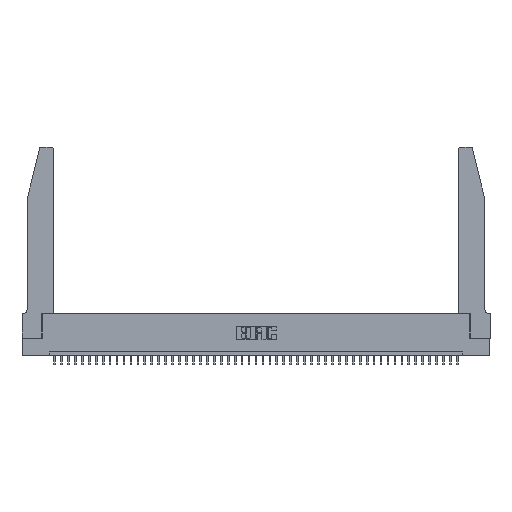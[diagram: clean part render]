
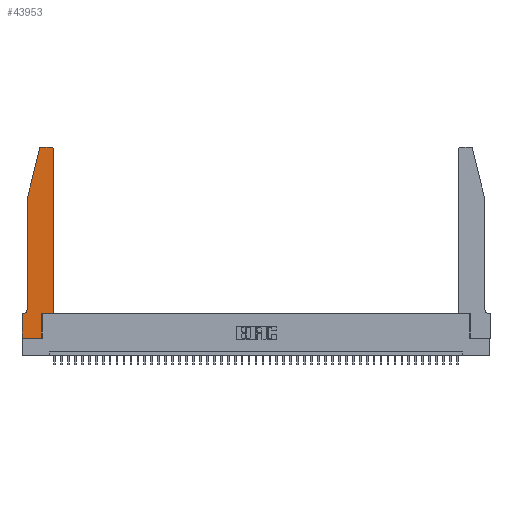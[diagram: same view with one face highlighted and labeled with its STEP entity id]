
A CAD part, top view. The second image highlights one B-rep face of the part: STEP entity #43953.
In plain terms, the highlighted planar face has unit normal (0, 0, 1).
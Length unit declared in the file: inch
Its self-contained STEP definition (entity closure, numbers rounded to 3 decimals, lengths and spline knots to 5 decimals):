
#138 = DIRECTION ( 'NONE',  ( -0.239, -0.971, 0. ) ) ;
#844 = DIRECTION ( 'NONE',  ( 1., 0., 0. ) ) ;
#2075 = VERTEX_POINT ( 'NONE', #14113 ) ;
#2103 = CARTESIAN_POINT ( 'NONE',  ( 0.284, 2.75, 0.37 ) ) ;
#2843 = VERTEX_POINT ( 'NONE', #15845 ) ;
#3227 = CARTESIAN_POINT ( 'NONE',  ( 0.4205, 2.72, 0.37 ) ) ;
#4551 = EDGE_CURVE ( 'NONE', #30048, #42664, #26186, .T. ) ;
#4882 = DIRECTION ( 'NONE',  ( 1., 0., 0. ) ) ;
#4928 = DIRECTION ( 'NONE',  ( 1., 0., 0. ) ) ;
#5244 = CARTESIAN_POINT ( 'NONE',  ( 0.2605, 2.75, 0.37 ) ) ;
#5633 = LINE ( 'NONE', #37370, #14106 ) ;
#5967 = VERTEX_POINT ( 'NONE', #39634 ) ;
#6289 = ORIENTED_EDGE ( 'NONE', *, *, #19652, .T. ) ;
#6685 = LINE ( 'NONE', #18117, #32146 ) ;
#7020 = EDGE_CURVE ( 'NONE', #42664, #39795, #6685, .T. ) ;
#8033 = CARTESIAN_POINT ( 'NONE',  ( 0.25487, 2.72718, 0.37 ) ) ;
#8486 = CARTESIAN_POINT ( 'NONE',  ( 0.0755, 2., 0.37 ) ) ;
#8851 = PLANE ( 'NONE',  #11352 ) ;
#10525 = EDGE_LOOP ( 'NONE', ( #17833, #34712, #24384, #11935, #15314, #38616, #31640, #6289, #16510, #16528, #33761, #29698 ) ) ;
#11204 = DIRECTION ( 'NONE',  ( -1., 0., 0. ) ) ;
#11352 = AXIS2_PLACEMENT_3D ( 'NONE', #44620, #30682, #4928 ) ;
#11652 = CIRCLE ( 'NONE', #34607, 0.07 ) ;
#11935 = ORIENTED_EDGE ( 'NONE', *, *, #13760, .T. ) ;
#12377 = LINE ( 'NONE', #18915, #35576 ) ;
#12575 = CARTESIAN_POINT ( 'NONE',  ( 0.0755, 0.42, 0.37 ) ) ;
#13193 = VERTEX_POINT ( 'NONE', #12575 ) ;
#13651 = DIRECTION ( 'NONE',  ( 1., 0., 0. ) ) ;
#13760 = EDGE_CURVE ( 'NONE', #39795, #13193, #5633, .T. ) ;
#14106 = VECTOR ( 'NONE', #18997, 39.37008 ) ;
#14113 = CARTESIAN_POINT ( 'NONE',  ( 0.4505, 0.35, 0.37 ) ) ;
#14118 = DIRECTION ( 'NONE',  ( 0., 0., 1. ) ) ;
#15143 = CARTESIAN_POINT ( 'NONE',  ( 0.0055, 0.42, 0.37 ) ) ;
#15176 = VECTOR ( 'NONE', #4882, 39.37008 ) ;
#15314 = ORIENTED_EDGE ( 'NONE', *, *, #15980, .T. ) ;
#15817 = VECTOR ( 'NONE', #844, 39.37008 ) ;
#15845 = CARTESIAN_POINT ( 'NONE',  ( 0.4205, 2.75, 0.37 ) ) ;
#15980 = EDGE_CURVE ( 'NONE', #13193, #18984, #11652, .T. ) ;
#16022 = LINE ( 'NONE', #38674, #18848 ) ;
#16424 = DIRECTION ( 'NONE',  ( 0., -1., 0. ) ) ;
#16510 = ORIENTED_EDGE ( 'NONE', *, *, #34084, .T. ) ;
#16528 = ORIENTED_EDGE ( 'NONE', *, *, #36713, .T. ) ;
#17636 = EDGE_CURVE ( 'NONE', #30359, #25173, #23959, .T. ) ;
#17833 = ORIENTED_EDGE ( 'NONE', *, *, #22985, .T. ) ;
#18117 = CARTESIAN_POINT ( 'NONE',  ( 0.0755, 2., 0.37 ) ) ;
#18536 = LINE ( 'NONE', #26353, #40649 ) ;
#18786 = DIRECTION ( 'NONE',  ( 0., 0., -1. ) ) ;
#18848 = VECTOR ( 'NONE', #42311, 39.37008 ) ;
#18915 = CARTESIAN_POINT ( 'NONE',  ( 0.0755, 0.35, 0.37 ) ) ;
#18984 = VERTEX_POINT ( 'NONE', #43914 ) ;
#18997 = DIRECTION ( 'NONE',  ( 0., -1., 0. ) ) ;
#19612 = FACE_OUTER_BOUND ( 'NONE', #10525, .T. ) ;
#19652 = EDGE_CURVE ( 'NONE', #25173, #43913, #32821, .T. ) ;
#20571 = LINE ( 'NONE', #37133, #15176 ) ;
#22470 = CARTESIAN_POINT ( 'NONE',  ( 0., 0., 0.37 ) ) ;
#22602 = CARTESIAN_POINT ( 'NONE',  ( 0.2865, 0., 0.37 ) ) ;
#22985 = EDGE_CURVE ( 'NONE', #2843, #30048, #38957, .T. ) ;
#23959 = LINE ( 'NONE', #38150, #38688 ) ;
#24384 = ORIENTED_EDGE ( 'NONE', *, *, #7020, .T. ) ;
#24496 = AXIS2_PLACEMENT_3D ( 'NONE', #3227, #14118, #13651 ) ;
#25173 = VERTEX_POINT ( 'NONE', #42006 ) ;
#26154 = VERTEX_POINT ( 'NONE', #43650 ) ;
#26186 = CIRCLE ( 'NONE', #36513, 0.03 ) ;
#26353 = CARTESIAN_POINT ( 'NONE',  ( 0.4505, 0.35, 0.37 ) ) ;
#26474 = CIRCLE ( 'NONE', #24496, 0.03 ) ;
#26504 = DIRECTION ( 'NONE',  ( 0., 1., 0. ) ) ;
#29332 = EDGE_CURVE ( 'NONE', #2075, #5967, #18536, .T. ) ;
#29698 = ORIENTED_EDGE ( 'NONE', *, *, #46114, .T. ) ;
#30048 = VERTEX_POINT ( 'NONE', #2103 ) ;
#30359 = VERTEX_POINT ( 'NONE', #34524 ) ;
#30682 = DIRECTION ( 'NONE',  ( 0., 0., 1. ) ) ;
#31640 = ORIENTED_EDGE ( 'NONE', *, *, #17636, .T. ) ;
#32146 = VECTOR ( 'NONE', #138, 39.37008 ) ;
#32680 = VECTOR ( 'NONE', #44621, 39.37008 ) ;
#32821 = LINE ( 'NONE', #22470, #15817 ) ;
#33761 = ORIENTED_EDGE ( 'NONE', *, *, #29332, .T. ) ;
#34084 = EDGE_CURVE ( 'NONE', #43913, #26154, #16022, .T. ) ;
#34524 = CARTESIAN_POINT ( 'NONE',  ( 0., 0.35, 0.37 ) ) ;
#34607 = AXIS2_PLACEMENT_3D ( 'NONE', #15143, #18786, #11204 ) ;
#34712 = ORIENTED_EDGE ( 'NONE', *, *, #4551, .T. ) ;
#35539 = CARTESIAN_POINT ( 'NONE',  ( 0.284, 2.72, 0.37 ) ) ;
#35576 = VECTOR ( 'NONE', #44263, 39.37008 ) ;
#36513 = AXIS2_PLACEMENT_3D ( 'NONE', #35539, #42839, #43149 ) ;
#36713 = EDGE_CURVE ( 'NONE', #26154, #2075, #20571, .T. ) ;
#36771 = EDGE_CURVE ( 'NONE', #18984, #30359, #12377, .T. ) ;
#37133 = CARTESIAN_POINT ( 'NONE',  ( 0.4505, 0.35, 0.37 ) ) ;
#37370 = CARTESIAN_POINT ( 'NONE',  ( 0.0755, 2., 0.37 ) ) ;
#38150 = CARTESIAN_POINT ( 'NONE',  ( 0., 0., 0.37 ) ) ;
#38616 = ORIENTED_EDGE ( 'NONE', *, *, #36771, .T. ) ;
#38674 = CARTESIAN_POINT ( 'NONE',  ( 0.2865, 0.35, 0.37 ) ) ;
#38688 = VECTOR ( 'NONE', #16424, 39.37008 ) ;
#38957 = LINE ( 'NONE', #5244, #32680 ) ;
#39634 = CARTESIAN_POINT ( 'NONE',  ( 0.4505, 2.72, 0.37 ) ) ;
#39795 = VERTEX_POINT ( 'NONE', #8486 ) ;
#40649 = VECTOR ( 'NONE', #26504, 39.37008 ) ;
#42006 = CARTESIAN_POINT ( 'NONE',  ( 0., 0., 0.37 ) ) ;
#42311 = DIRECTION ( 'NONE',  ( 0., 1., 0. ) ) ;
#42664 = VERTEX_POINT ( 'NONE', #8033 ) ;
#42839 = DIRECTION ( 'NONE',  ( 0., 0., 1. ) ) ;
#43149 = DIRECTION ( 'NONE',  ( 1., 0., 0. ) ) ;
#43650 = CARTESIAN_POINT ( 'NONE',  ( 0.2865, 0.35, 0.37 ) ) ;
#43913 = VERTEX_POINT ( 'NONE', #22602 ) ;
#43914 = CARTESIAN_POINT ( 'NONE',  ( 0.0055, 0.35, 0.37 ) ) ;
#43953 = ADVANCED_FACE ( 'NONE', ( #19612 ), #8851, .T. ) ;
#44263 = DIRECTION ( 'NONE',  ( -1., 0., 0. ) ) ;
#44620 = CARTESIAN_POINT ( 'NONE',  ( 0., 0.35, 0.37 ) ) ;
#44621 = DIRECTION ( 'NONE',  ( -1., 0., 0. ) ) ;
#46114 = EDGE_CURVE ( 'NONE', #5967, #2843, #26474, .T. ) ;
